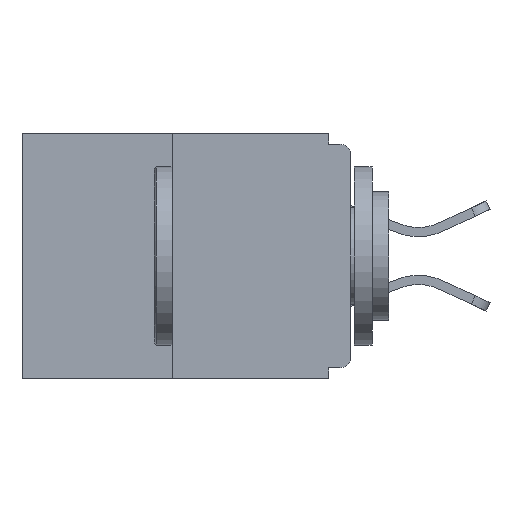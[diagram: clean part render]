
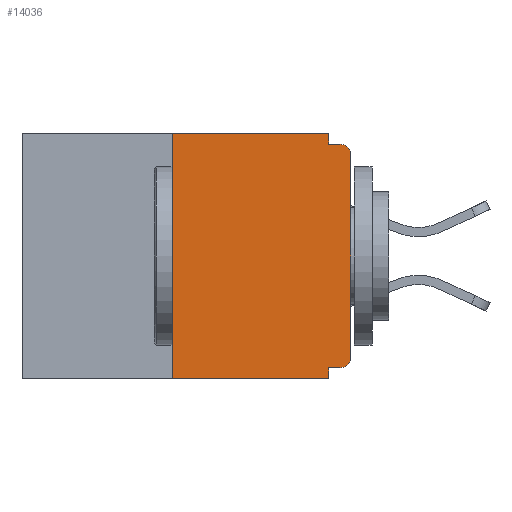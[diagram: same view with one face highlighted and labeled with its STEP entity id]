
A CAD part, left-side view. The second image highlights one B-rep face of the part: STEP entity #14036.
In plain terms, the highlighted planar face has unit normal (-1, 0, 0).
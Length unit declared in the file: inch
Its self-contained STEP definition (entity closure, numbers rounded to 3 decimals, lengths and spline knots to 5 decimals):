
#257 = VECTOR ( 'NONE', #13431, 39.37008 ) ;
#262 = ORIENTED_EDGE ( 'NONE', *, *, #10043, .T. ) ;
#573 = DIRECTION ( 'NONE',  ( 1., 0., 0. ) ) ;
#670 = DIRECTION ( 'NONE',  ( 0., 0., -1. ) ) ;
#970 = CARTESIAN_POINT ( 'NONE',  ( 0., 0.015, -0.015 ) ) ;
#1164 = EDGE_CURVE ( 'NONE', #4068, #4328, #3272, .T. ) ;
#1247 = CARTESIAN_POINT ( 'NONE',  ( 0., 0.25, 0. ) ) ;
#1359 = DIRECTION ( 'NONE',  ( 0., 0., -1. ) ) ;
#1392 = VECTOR ( 'NONE', #1359, 39.37008 ) ;
#1491 = DIRECTION ( 'NONE',  ( 0., 0., -1. ) ) ;
#1722 = PLANE ( 'NONE',  #10278 ) ;
#2515 = DIRECTION ( 'NONE',  ( -1., 0., 0. ) ) ;
#2999 = ORIENTED_EDGE ( 'NONE', *, *, #1164, .T. ) ;
#3170 = LINE ( 'NONE', #4309, #8143 ) ;
#3272 = CIRCLE ( 'NONE', #3488, 0.015 ) ;
#3383 = DIRECTION ( 'NONE',  ( 0., 0., 1. ) ) ;
#3488 = AXIS2_PLACEMENT_3D ( 'NONE', #12169, #5516, #5656 ) ;
#3855 = VERTEX_POINT ( 'NONE', #7365 ) ;
#3902 = CARTESIAN_POINT ( 'NONE',  ( 0., 0.031, 0. ) ) ;
#3955 = VECTOR ( 'NONE', #8513, 39.37008 ) ;
#3997 = EDGE_CURVE ( 'NONE', #9358, #8780, #12727, .T. ) ;
#4012 = LINE ( 'NONE', #4891, #7767 ) ;
#4068 = VERTEX_POINT ( 'NONE', #7614 ) ;
#4119 = VECTOR ( 'NONE', #3383, 39.37008 ) ;
#4309 = CARTESIAN_POINT ( 'NONE',  ( 0., 0., -0.015 ) ) ;
#4328 = VERTEX_POINT ( 'NONE', #970 ) ;
#4793 = EDGE_CURVE ( 'NONE', #8780, #7075, #11155, .T. ) ;
#4891 = CARTESIAN_POINT ( 'NONE',  ( 0., 0.46, -0.343 ) ) ;
#5516 = DIRECTION ( 'NONE',  ( -1., 0., 0. ) ) ;
#5656 = DIRECTION ( 'NONE',  ( 0., 0., -1. ) ) ;
#5757 = CARTESIAN_POINT ( 'NONE',  ( 0., 0., -0.313 ) ) ;
#5976 = ORIENTED_EDGE ( 'NONE', *, *, #13021, .T. ) ;
#6178 = DIRECTION ( 'NONE',  ( 0., -1., 0. ) ) ;
#6523 = EDGE_CURVE ( 'NONE', #12352, #7746, #9554, .T. ) ;
#6835 = LINE ( 'NONE', #9479, #3955 ) ;
#7041 = CARTESIAN_POINT ( 'NONE',  ( 0., 0.015, -0.313 ) ) ;
#7075 = VERTEX_POINT ( 'NONE', #10466 ) ;
#7095 = CARTESIAN_POINT ( 'NONE',  ( 0., 0., -0.328 ) ) ;
#7197 = CARTESIAN_POINT ( 'NONE',  ( 0., 0.46, 0. ) ) ;
#7333 = FACE_OUTER_BOUND ( 'NONE', #7966, .T. ) ;
#7365 = CARTESIAN_POINT ( 'NONE',  ( 0., 0.25, -0.343 ) ) ;
#7567 = VECTOR ( 'NONE', #8115, 39.37008 ) ;
#7614 = CARTESIAN_POINT ( 'NONE',  ( 0., 0., -0.03 ) ) ;
#7746 = VERTEX_POINT ( 'NONE', #10015 ) ;
#7767 = VECTOR ( 'NONE', #6178, 39.37008 ) ;
#7925 = ORIENTED_EDGE ( 'NONE', *, *, #4793, .F. ) ;
#7966 = EDGE_LOOP ( 'NONE', ( #9700, #9504, #262, #12216, #8681, #11439, #5976, #2999, #13346, #7925 ) ) ;
#8115 = DIRECTION ( 'NONE',  ( 0., 0., -1. ) ) ;
#8143 = VECTOR ( 'NONE', #11936, 39.37008 ) ;
#8513 = DIRECTION ( 'NONE',  ( 0., 0., 1. ) ) ;
#8546 = EDGE_CURVE ( 'NONE', #7075, #4328, #3170, .T. ) ;
#8648 = VECTOR ( 'NONE', #12077, 39.37008 ) ;
#8681 = ORIENTED_EDGE ( 'NONE', *, *, #11312, .F. ) ;
#8780 = VERTEX_POINT ( 'NONE', #13600 ) ;
#9358 = VERTEX_POINT ( 'NONE', #12040 ) ;
#9384 = VERTEX_POINT ( 'NONE', #12090 ) ;
#9479 = CARTESIAN_POINT ( 'NONE',  ( 0., 0., 0. ) ) ;
#9504 = ORIENTED_EDGE ( 'NONE', *, *, #12555, .F. ) ;
#9554 = LINE ( 'NONE', #11600, #1392 ) ;
#9700 = ORIENTED_EDGE ( 'NONE', *, *, #3997, .F. ) ;
#9748 = VERTEX_POINT ( 'NONE', #5757 ) ;
#9756 = EDGE_CURVE ( 'NONE', #9384, #9748, #13563, .T. ) ;
#10015 = CARTESIAN_POINT ( 'NONE',  ( 0., 0.031, -0.343 ) ) ;
#10043 = EDGE_CURVE ( 'NONE', #3855, #7746, #4012, .T. ) ;
#10107 = LINE ( 'NONE', #1247, #4119 ) ;
#10278 = AXIS2_PLACEMENT_3D ( 'NONE', #7197, #573, #670 ) ;
#10330 = LINE ( 'NONE', #7095, #257 ) ;
#10466 = CARTESIAN_POINT ( 'NONE',  ( 0., 0.031, -0.015 ) ) ;
#10952 = CARTESIAN_POINT ( 'NONE',  ( 0., 0.46, 0. ) ) ;
#11155 = LINE ( 'NONE', #3902, #7567 ) ;
#11312 = EDGE_CURVE ( 'NONE', #9384, #12352, #10330, .T. ) ;
#11439 = ORIENTED_EDGE ( 'NONE', *, *, #9756, .T. ) ;
#11600 = CARTESIAN_POINT ( 'NONE',  ( 0., 0.031, -0.343 ) ) ;
#11614 = AXIS2_PLACEMENT_3D ( 'NONE', #7041, #2515, #1491 ) ;
#11936 = DIRECTION ( 'NONE',  ( 0., -1., 0. ) ) ;
#12040 = CARTESIAN_POINT ( 'NONE',  ( 0., 0.25, 0. ) ) ;
#12077 = DIRECTION ( 'NONE',  ( 0., -1., 0. ) ) ;
#12090 = CARTESIAN_POINT ( 'NONE',  ( 0., 0.015, -0.328 ) ) ;
#12169 = CARTESIAN_POINT ( 'NONE',  ( 0., 0.015, -0.03 ) ) ;
#12216 = ORIENTED_EDGE ( 'NONE', *, *, #6523, .F. ) ;
#12352 = VERTEX_POINT ( 'NONE', #13790 ) ;
#12555 = EDGE_CURVE ( 'NONE', #3855, #9358, #10107, .T. ) ;
#12727 = LINE ( 'NONE', #10952, #8648 ) ;
#13021 = EDGE_CURVE ( 'NONE', #9748, #4068, #6835, .T. ) ;
#13346 = ORIENTED_EDGE ( 'NONE', *, *, #8546, .F. ) ;
#13431 = DIRECTION ( 'NONE',  ( 0., 1., 0. ) ) ;
#13563 = CIRCLE ( 'NONE', #11614, 0.015 ) ;
#13600 = CARTESIAN_POINT ( 'NONE',  ( 0., 0.031, 0. ) ) ;
#13790 = CARTESIAN_POINT ( 'NONE',  ( 0., 0.031, -0.328 ) ) ;
#14036 = ADVANCED_FACE ( 'NONE', ( #7333 ), #1722, .F. ) ;
